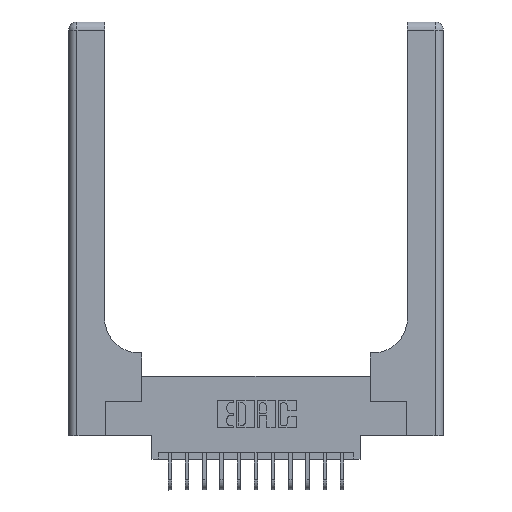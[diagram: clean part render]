
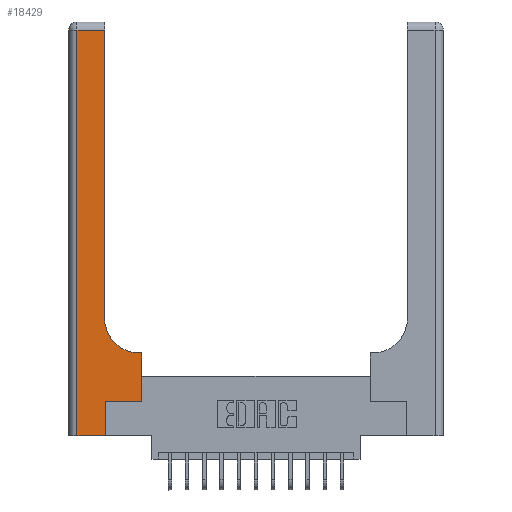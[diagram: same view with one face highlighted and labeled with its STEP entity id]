
A CAD part, top view. The second image highlights one B-rep face of the part: STEP entity #18429.
In plain terms, the highlighted planar face has unit normal (0, 0, 1).
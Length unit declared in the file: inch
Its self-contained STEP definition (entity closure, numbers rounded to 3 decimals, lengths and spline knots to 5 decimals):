
#94 = CARTESIAN_POINT ( 'NONE',  ( 0.528, 0.25, 0.37 ) ) ;
#562 = VECTOR ( 'NONE', #2409, 39.37008 ) ;
#1125 = DIRECTION ( 'NONE',  ( 1., 0., 0. ) ) ;
#1449 = CARTESIAN_POINT ( 'NONE',  ( 0.265, 0.25, 0.37 ) ) ;
#1558 = CARTESIAN_POINT ( 'NONE',  ( 0., 0., 0.37 ) ) ;
#2409 = DIRECTION ( 'NONE',  ( 0., 1., 0. ) ) ;
#2463 = EDGE_CURVE ( 'NONE', #4428, #11642, #9211, .T. ) ;
#3339 = EDGE_CURVE ( 'NONE', #12407, #6939, #9349, .T. ) ;
#3390 = VECTOR ( 'NONE', #13602, 39.37008 ) ;
#3619 = CARTESIAN_POINT ( 'NONE',  ( 0.26, 2.94, 0.37 ) ) ;
#3890 = VERTEX_POINT ( 'NONE', #17576 ) ;
#4051 = VERTEX_POINT ( 'NONE', #12453 ) ;
#4428 = VERTEX_POINT ( 'NONE', #3619 ) ;
#4603 = PLANE ( 'NONE',  #9861 ) ;
#4702 = DIRECTION ( 'NONE',  ( -1., 0., 0. ) ) ;
#4753 = ORIENTED_EDGE ( 'NONE', *, *, #12262, .T. ) ;
#4881 = ORIENTED_EDGE ( 'NONE', *, *, #9038, .T. ) ;
#5760 = ORIENTED_EDGE ( 'NONE', *, *, #5982, .T. ) ;
#5896 = LINE ( 'NONE', #11784, #12429 ) ;
#5982 = EDGE_CURVE ( 'NONE', #11642, #4051, #6376, .T. ) ;
#6376 = LINE ( 'NONE', #6561, #7896 ) ;
#6546 = EDGE_CURVE ( 'NONE', #6945, #12278, #11381, .T. ) ;
#6561 = CARTESIAN_POINT ( 'NONE',  ( 0.06, 3., 0.37 ) ) ;
#6939 = VERTEX_POINT ( 'NONE', #1449 ) ;
#6945 = VERTEX_POINT ( 'NONE', #10215 ) ;
#7768 = AXIS2_PLACEMENT_3D ( 'NONE', #14473, #11601, #11410 ) ;
#7800 = CARTESIAN_POINT ( 'NONE',  ( 0.265, 0., 0.37 ) ) ;
#7896 = VECTOR ( 'NONE', #16879, 39.37008 ) ;
#8001 = CARTESIAN_POINT ( 'NONE',  ( 0.265, 0., 0.37 ) ) ;
#8442 = LINE ( 'NONE', #14235, #17444 ) ;
#8562 = EDGE_CURVE ( 'NONE', #3890, #17003, #16588, .T. ) ;
#8763 = CARTESIAN_POINT ( 'NONE',  ( 0.26, 0.6, 0.37 ) ) ;
#9038 = EDGE_CURVE ( 'NONE', #4051, #12407, #10583, .T. ) ;
#9211 = LINE ( 'NONE', #15026, #3390 ) ;
#9349 = LINE ( 'NONE', #8001, #562 ) ;
#9446 = ORIENTED_EDGE ( 'NONE', *, *, #8562, .T. ) ;
#9861 = AXIS2_PLACEMENT_3D ( 'NONE', #11954, #17804, #4702 ) ;
#10215 = CARTESIAN_POINT ( 'NONE',  ( 0.528, 0.25, 0.37 ) ) ;
#10283 = LINE ( 'NONE', #8763, #16023 ) ;
#10386 = CARTESIAN_POINT ( 'NONE',  ( 0.528, 0.6, 0.37 ) ) ;
#10583 = LINE ( 'NONE', #1558, #11436 ) ;
#10969 = EDGE_LOOP ( 'NONE', ( #4753, #11141, #5760, #4881, #13137, #17700, #14198, #16628, #9446 ) ) ;
#11095 = EDGE_CURVE ( 'NONE', #12278, #3890, #10283, .T. ) ;
#11141 = ORIENTED_EDGE ( 'NONE', *, *, #2463, .T. ) ;
#11381 = LINE ( 'NONE', #94, #11829 ) ;
#11410 = DIRECTION ( 'NONE',  ( 1., 0., 0. ) ) ;
#11436 = VECTOR ( 'NONE', #11723, 39.37008 ) ;
#11467 = DIRECTION ( 'NONE',  ( 0., 1., 0. ) ) ;
#11601 = DIRECTION ( 'NONE',  ( 0., 0., -1. ) ) ;
#11642 = VERTEX_POINT ( 'NONE', #11854 ) ;
#11707 = DIRECTION ( 'NONE',  ( 0., 1., 0. ) ) ;
#11723 = DIRECTION ( 'NONE',  ( 1., 0., 0. ) ) ;
#11784 = CARTESIAN_POINT ( 'NONE',  ( 0.26, 3., 0.37 ) ) ;
#11829 = VECTOR ( 'NONE', #11467, 39.37008 ) ;
#11854 = CARTESIAN_POINT ( 'NONE',  ( 0.06, 2.94, 0.37 ) ) ;
#11954 = CARTESIAN_POINT ( 'NONE',  ( 0., 3., 0.37 ) ) ;
#12218 = FACE_OUTER_BOUND ( 'NONE', #10969, .T. ) ;
#12262 = EDGE_CURVE ( 'NONE', #17003, #4428, #5896, .T. ) ;
#12278 = VERTEX_POINT ( 'NONE', #10386 ) ;
#12407 = VERTEX_POINT ( 'NONE', #7800 ) ;
#12429 = VECTOR ( 'NONE', #11707, 39.37008 ) ;
#12453 = CARTESIAN_POINT ( 'NONE',  ( 0.06, 0., 0.37 ) ) ;
#13137 = ORIENTED_EDGE ( 'NONE', *, *, #3339, .T. ) ;
#13602 = DIRECTION ( 'NONE',  ( -1., 0., 0. ) ) ;
#14013 = CARTESIAN_POINT ( 'NONE',  ( 0.26, 0.85, 0.37 ) ) ;
#14198 = ORIENTED_EDGE ( 'NONE', *, *, #6546, .T. ) ;
#14235 = CARTESIAN_POINT ( 'NONE',  ( 0.265, 0.25, 0.37 ) ) ;
#14473 = CARTESIAN_POINT ( 'NONE',  ( 0.51, 0.85, 0.37 ) ) ;
#14565 = DIRECTION ( 'NONE',  ( -1., 0., 0. ) ) ;
#15026 = CARTESIAN_POINT ( 'NONE',  ( 0., 2.94, 0.37 ) ) ;
#16023 = VECTOR ( 'NONE', #14565, 39.37008 ) ;
#16588 = CIRCLE ( 'NONE', #7768, 0.25 ) ;
#16628 = ORIENTED_EDGE ( 'NONE', *, *, #11095, .T. ) ;
#16879 = DIRECTION ( 'NONE',  ( 0., -1., 0. ) ) ;
#17003 = VERTEX_POINT ( 'NONE', #14013 ) ;
#17444 = VECTOR ( 'NONE', #1125, 39.37008 ) ;
#17576 = CARTESIAN_POINT ( 'NONE',  ( 0.51, 0.6, 0.37 ) ) ;
#17700 = ORIENTED_EDGE ( 'NONE', *, *, #18661, .T. ) ;
#17804 = DIRECTION ( 'NONE',  ( 0., 0., -1. ) ) ;
#18429 = ADVANCED_FACE ( 'NONE', ( #12218 ), #4603, .F. ) ;
#18661 = EDGE_CURVE ( 'NONE', #6939, #6945, #8442, .T. ) ;
